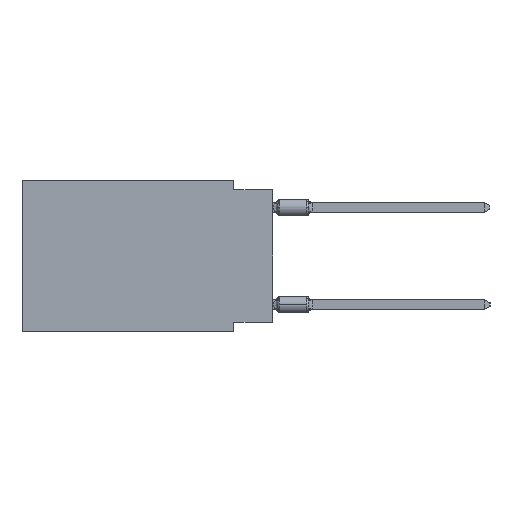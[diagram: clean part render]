
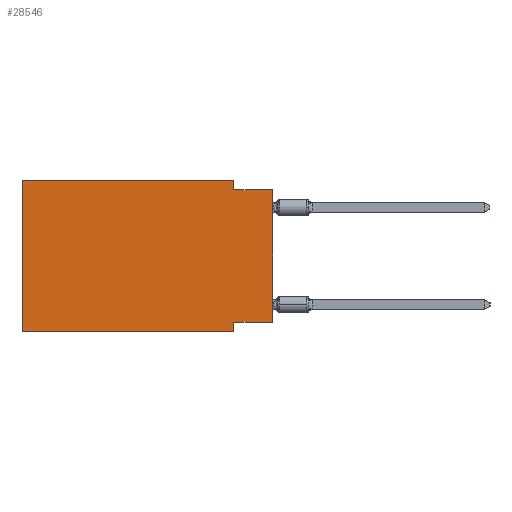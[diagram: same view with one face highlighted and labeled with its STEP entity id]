
A CAD part, left-side view. The second image highlights one B-rep face of the part: STEP entity #28546.
In plain terms, the highlighted planar face has unit normal (-1, 0, 0).
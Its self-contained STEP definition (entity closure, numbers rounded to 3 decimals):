
#91 = PLANE ( 'NONE',  #41439 ) ;
#528 = VECTOR ( 'NONE', #15814, 1000. ) ;
#846 = CARTESIAN_POINT ( 'NONE',  ( 0., 16.383, -9.906 ) ) ;
#1391 = CARTESIAN_POINT ( 'NONE',  ( 0., 0., -9.271 ) ) ;
#2020 = VERTEX_POINT ( 'NONE', #846 ) ;
#2115 = CARTESIAN_POINT ( 'NONE',  ( 0., 0., -9.271 ) ) ;
#2213 = CARTESIAN_POINT ( 'NONE',  ( 0., 2.54, 0. ) ) ;
#3025 = VECTOR ( 'NONE', #20780, 1000. ) ;
#3826 = DIRECTION ( 'NONE',  ( 0., 0., 1. ) ) ;
#4296 = ORIENTED_EDGE ( 'NONE', *, *, #25425, .F. ) ;
#5005 = LINE ( 'NONE', #2213, #8642 ) ;
#5828 = VERTEX_POINT ( 'NONE', #40659 ) ;
#6044 = LINE ( 'NONE', #19129, #18101 ) ;
#6156 = CARTESIAN_POINT ( 'NONE',  ( 0., 2.54, -9.906 ) ) ;
#7822 = EDGE_CURVE ( 'NONE', #2020, #5828, #23547, .T. ) ;
#7895 = LINE ( 'NONE', #40294, #10874 ) ;
#8216 = DIRECTION ( 'NONE',  ( 0., 0., -1. ) ) ;
#8642 = VECTOR ( 'NONE', #8216, 1000. ) ;
#9041 = DIRECTION ( 'NONE',  ( 0., -1., 0. ) ) ;
#9402 = CARTESIAN_POINT ( 'NONE',  ( 0., 0., 0. ) ) ;
#10006 = ORIENTED_EDGE ( 'NONE', *, *, #37129, .F. ) ;
#10400 = VECTOR ( 'NONE', #26104, 1000. ) ;
#10874 = VECTOR ( 'NONE', #36859, 1000. ) ;
#11483 = LINE ( 'NONE', #34658, #16941 ) ;
#12718 = CARTESIAN_POINT ( 'NONE',  ( 0., 2.54, 0. ) ) ;
#12892 = CARTESIAN_POINT ( 'NONE',  ( 0., 2.54, -9.271 ) ) ;
#14415 = ORIENTED_EDGE ( 'NONE', *, *, #20386, .T. ) ;
#14588 = EDGE_LOOP ( 'NONE', ( #14415, #27929, #30211, #10006, #28631, #33947, #27977, #4296 ) ) ;
#15419 = LINE ( 'NONE', #9402, #10400 ) ;
#15814 = DIRECTION ( 'NONE',  ( 0., 0., -1. ) ) ;
#16435 = VECTOR ( 'NONE', #3826, 1000. ) ;
#16941 = VECTOR ( 'NONE', #30788, 1000. ) ;
#18055 = CARTESIAN_POINT ( 'NONE',  ( 0., 2.54, -0.635 ) ) ;
#18101 = VECTOR ( 'NONE', #9041, 1000. ) ;
#19035 = LINE ( 'NONE', #6156, #528 ) ;
#19129 = CARTESIAN_POINT ( 'NONE',  ( 0., 16.383, -9.906 ) ) ;
#19408 = CARTESIAN_POINT ( 'NONE',  ( 0., 16.383, 0. ) ) ;
#19808 = FACE_OUTER_BOUND ( 'NONE', #14588, .T. ) ;
#20386 = EDGE_CURVE ( 'NONE', #22224, #32853, #15419, .T. ) ;
#20569 = CARTESIAN_POINT ( 'NONE',  ( 0., 0., -0.635 ) ) ;
#20780 = DIRECTION ( 'NONE',  ( 0., 1., 0. ) ) ;
#22224 = VERTEX_POINT ( 'NONE', #1391 ) ;
#22774 = EDGE_CURVE ( 'NONE', #2020, #24614, #6044, .T. ) ;
#23547 = LINE ( 'NONE', #29356, #16435 ) ;
#24614 = VERTEX_POINT ( 'NONE', #33819 ) ;
#25170 = VERTEX_POINT ( 'NONE', #12892 ) ;
#25425 = EDGE_CURVE ( 'NONE', #22224, #25170, #27644, .T. ) ;
#26104 = DIRECTION ( 'NONE',  ( 0., 0., 1. ) ) ;
#27644 = LINE ( 'NONE', #2115, #3025 ) ;
#27929 = ORIENTED_EDGE ( 'NONE', *, *, #38894, .F. ) ;
#27977 = ORIENTED_EDGE ( 'NONE', *, *, #35740, .F. ) ;
#28546 = ADVANCED_FACE ( 'NONE', ( #19808 ), #91, .F. ) ;
#28631 = ORIENTED_EDGE ( 'NONE', *, *, #7822, .F. ) ;
#29356 = CARTESIAN_POINT ( 'NONE',  ( 0., 16.383, 0. ) ) ;
#30014 = EDGE_CURVE ( 'NONE', #37733, #31232, #5005, .T. ) ;
#30211 = ORIENTED_EDGE ( 'NONE', *, *, #30014, .F. ) ;
#30788 = DIRECTION ( 'NONE',  ( 0., -1., 0. ) ) ;
#31232 = VERTEX_POINT ( 'NONE', #18055 ) ;
#32853 = VERTEX_POINT ( 'NONE', #20569 ) ;
#33819 = CARTESIAN_POINT ( 'NONE',  ( 0., 2.54, -9.906 ) ) ;
#33947 = ORIENTED_EDGE ( 'NONE', *, *, #22774, .T. ) ;
#34658 = CARTESIAN_POINT ( 'NONE',  ( 0., 16.383, 0. ) ) ;
#35740 = EDGE_CURVE ( 'NONE', #25170, #24614, #19035, .T. ) ;
#36859 = DIRECTION ( 'NONE',  ( 0., -1., 0. ) ) ;
#37129 = EDGE_CURVE ( 'NONE', #5828, #37733, #11483, .T. ) ;
#37733 = VERTEX_POINT ( 'NONE', #12718 ) ;
#38727 = DIRECTION ( 'NONE',  ( 0., 0., -1. ) ) ;
#38894 = EDGE_CURVE ( 'NONE', #31232, #32853, #7895, .T. ) ;
#38934 = DIRECTION ( 'NONE',  ( 1., 0., 0. ) ) ;
#40294 = CARTESIAN_POINT ( 'NONE',  ( 0., 0., -0.635 ) ) ;
#40659 = CARTESIAN_POINT ( 'NONE',  ( 0., 16.383, 0. ) ) ;
#41439 = AXIS2_PLACEMENT_3D ( 'NONE', #19408, #38934, #38727 ) ;
